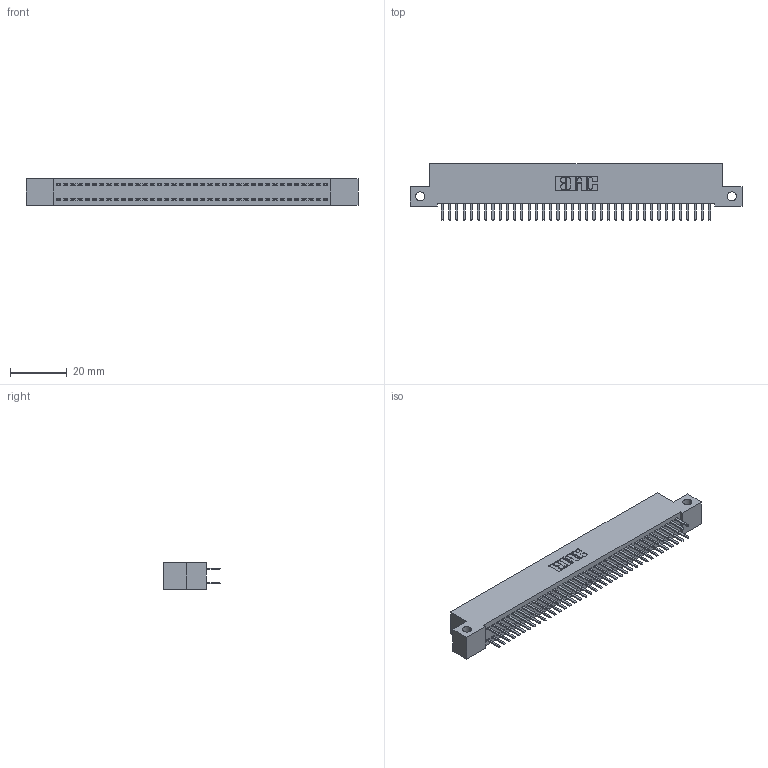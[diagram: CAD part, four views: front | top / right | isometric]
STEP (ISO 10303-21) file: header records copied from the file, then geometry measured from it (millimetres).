
FILE_DESCRIPTION (( 'STEP AP203' ), '1' );
FILE_NAME ('342-076-520-212.STEP', '2019-10-03T17:40:58', ( '' ), ( '' ), 'SwSTEP 2.0', 'SolidWorks 2016', '' );
FILE_SCHEMA (( 'CONFIG_CONTROL_DESIGN' ));
Length unit declared in the file: inch
Products named in the file (3): 342-076-520-212; 342 Part_Side Mount; 345-292-001_345-293-120
Assembly tree (77 placements, depth 2):
  342-076-520-212
    342 Part_Side Mount
    345-292-001_345-293-120  x76
Bounding box: 116.84 x 20.02 x 9.4 mm (x, y, z)
Volume: 10371.8 mm3; surface area: 16545.5 mm2
Topology: 77 solids, 77 shells, 4366 faces, 12687 edges, 8254 vertices
Faces by surface type: plane 2954, cylinder 1412
Entity records: 24949 total; most frequent: CARTESIAN_POINT 4150, ORIENTED_EDGE 4074, DIRECTION 3541, EDGE_CURVE 2037, VECTOR 1905, LINE 1905, VERTEX_POINT 1354, AXIS2_PLACEMENT_3D 818
